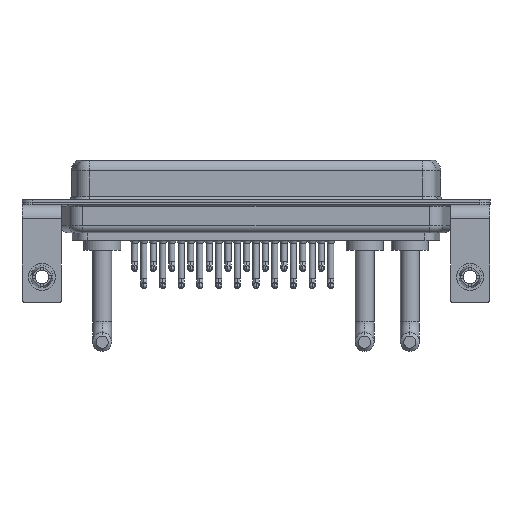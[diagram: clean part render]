
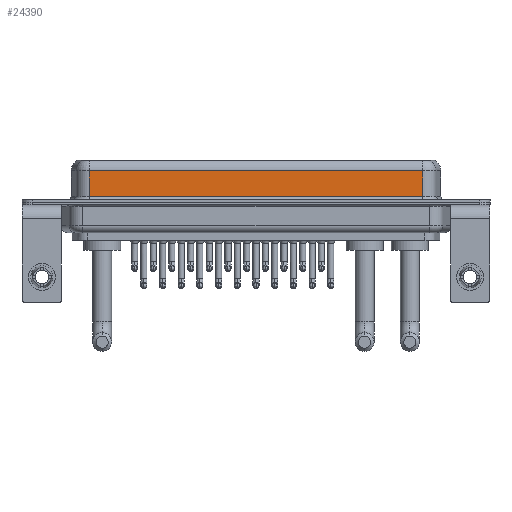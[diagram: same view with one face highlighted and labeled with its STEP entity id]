
A CAD part, front view. The second image highlights one B-rep face of the part: STEP entity #24390.
In plain terms, the highlighted planar face has unit normal (0, -1, 0).
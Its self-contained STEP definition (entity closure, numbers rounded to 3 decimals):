
#92 = ORIENTED_EDGE ( 'NONE', *, *, #13683, .F. ) ;
#932 = CARTESIAN_POINT ( 'NONE',  ( 56.462, -3.95, 4.65 ) ) ;
#2490 = LINE ( 'NONE', #10585, #9726 ) ;
#2621 = CARTESIAN_POINT ( 'NONE',  ( 7.038, -3.95, 6.4 ) ) ;
#2970 = DIRECTION ( 'NONE',  ( 0., 1., 0. ) ) ;
#3751 = EDGE_CURVE ( 'NONE', #21574, #23575, #4757, .T. ) ;
#4324 = VECTOR ( 'NONE', #12950, 1000. ) ;
#4576 = EDGE_LOOP ( 'NONE', ( #92, #9880, #15913, #10595 ) ) ;
#4757 = LINE ( 'NONE', #2621, #17872 ) ;
#4854 = CARTESIAN_POINT ( 'NONE',  ( 56.462, -3.95, 4.65 ) ) ;
#4973 = CARTESIAN_POINT ( 'NONE',  ( 56.462, -3.95, 6.4 ) ) ;
#5019 = DIRECTION ( 'NONE',  ( 0., 0., -1. ) ) ;
#6964 = FACE_OUTER_BOUND ( 'NONE', #4576, .T. ) ;
#7015 = DIRECTION ( 'NONE',  ( 1., 0., 0. ) ) ;
#7452 = VERTEX_POINT ( 'NONE', #14627 ) ;
#8503 = CARTESIAN_POINT ( 'NONE',  ( 56.462, -3.95, 0.9 ) ) ;
#9726 = VECTOR ( 'NONE', #5019, 1000. ) ;
#9880 = ORIENTED_EDGE ( 'NONE', *, *, #22506, .T. ) ;
#10585 = CARTESIAN_POINT ( 'NONE',  ( 56.462, -3.95, 6.4 ) ) ;
#10595 = ORIENTED_EDGE ( 'NONE', *, *, #23331, .T. ) ;
#11068 = DIRECTION ( 'NONE',  ( 0., 0., 1. ) ) ;
#11866 = VERTEX_POINT ( 'NONE', #932 ) ;
#12950 = DIRECTION ( 'NONE',  ( -1., 0., 0. ) ) ;
#13008 = CARTESIAN_POINT ( 'NONE',  ( 7.038, -3.95, 4.65 ) ) ;
#13683 = EDGE_CURVE ( 'NONE', #11866, #7452, #2490, .T. ) ;
#14319 = DIRECTION ( 'NONE',  ( 0., 0., -1. ) ) ;
#14484 = LINE ( 'NONE', #8503, #19574 ) ;
#14627 = CARTESIAN_POINT ( 'NONE',  ( 56.462, -3.95, 0.9 ) ) ;
#15412 = AXIS2_PLACEMENT_3D ( 'NONE', #4973, #2970, #11068 ) ;
#15913 = ORIENTED_EDGE ( 'NONE', *, *, #3751, .T. ) ;
#17872 = VECTOR ( 'NONE', #14319, 1000. ) ;
#19574 = VECTOR ( 'NONE', #7015, 1000. ) ;
#20999 = LINE ( 'NONE', #4854, #4324 ) ;
#21574 = VERTEX_POINT ( 'NONE', #13008 ) ;
#21813 = CARTESIAN_POINT ( 'NONE',  ( 7.038, -3.95, 0.9 ) ) ;
#22506 = EDGE_CURVE ( 'NONE', #11866, #21574, #20999, .T. ) ;
#23103 = PLANE ( 'NONE',  #15412 ) ;
#23331 = EDGE_CURVE ( 'NONE', #23575, #7452, #14484, .T. ) ;
#23575 = VERTEX_POINT ( 'NONE', #21813 ) ;
#24390 = ADVANCED_FACE ( 'NONE', ( #6964 ), #23103, .F. ) ;
